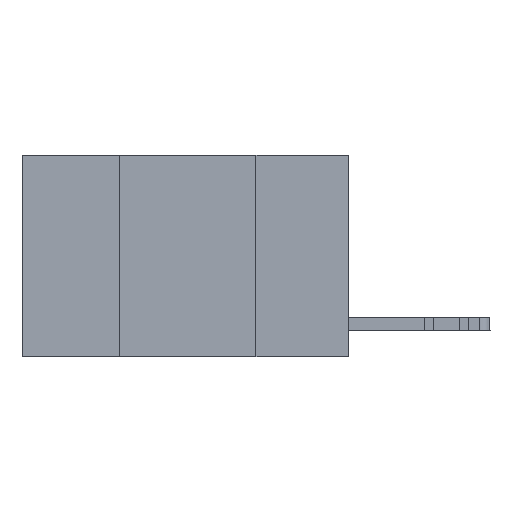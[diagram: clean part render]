
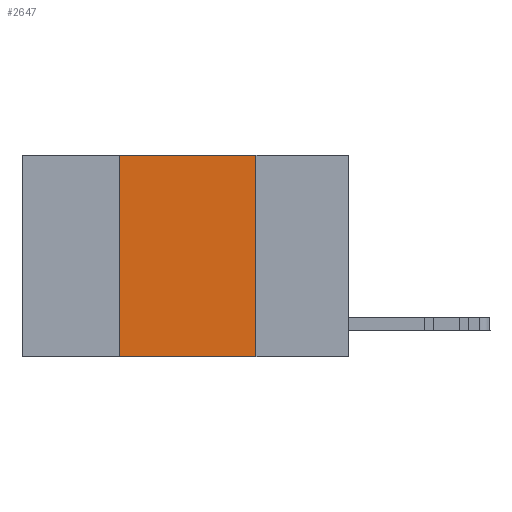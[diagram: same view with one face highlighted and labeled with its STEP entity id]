
A CAD part, left-side view. The second image highlights one B-rep face of the part: STEP entity #2647.
In plain terms, the highlighted planar face has unit normal (-1, 0, 0).
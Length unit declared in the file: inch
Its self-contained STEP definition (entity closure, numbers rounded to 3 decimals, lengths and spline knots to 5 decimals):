
#176 = PLANE ( 'NONE',  #8069 ) ;
#1855 = CARTESIAN_POINT ( 'NONE',  ( 0., 0.17, 0. ) ) ;
#2530 = CARTESIAN_POINT ( 'NONE',  ( 0., 0.6, 0. ) ) ;
#2647 = ADVANCED_FACE ( 'NONE', ( #24668 ), #176, .F. ) ;
#3897 = ORIENTED_EDGE ( 'NONE', *, *, #20488, .F. ) ;
#4731 = DIRECTION ( 'NONE',  ( 1., 0., 0. ) ) ;
#4996 = ORIENTED_EDGE ( 'NONE', *, *, #9708, .F. ) ;
#5467 = VECTOR ( 'NONE', #11132, 39.37008 ) ;
#7430 = VERTEX_POINT ( 'NONE', #26797 ) ;
#8069 = AXIS2_PLACEMENT_3D ( 'NONE', #2530, #4731, #24822 ) ;
#8283 = LINE ( 'NONE', #1855, #28602 ) ;
#8709 = DIRECTION ( 'NONE',  ( 0., 0., -1. ) ) ;
#9119 = VECTOR ( 'NONE', #28065, 39.37008 ) ;
#9708 = EDGE_CURVE ( 'NONE', #13549, #7430, #8283, .T. ) ;
#9821 = LINE ( 'NONE', #14484, #9119 ) ;
#10355 = CARTESIAN_POINT ( 'NONE',  ( 0., 0.42, 0. ) ) ;
#10970 = VERTEX_POINT ( 'NONE', #10355 ) ;
#11132 = DIRECTION ( 'NONE',  ( 0., 0., 1. ) ) ;
#11523 = VECTOR ( 'NONE', #23110, 39.37008 ) ;
#13015 = CARTESIAN_POINT ( 'NONE',  ( 0., 0.42, -0.37 ) ) ;
#13306 = ORIENTED_EDGE ( 'NONE', *, *, #21568, .F. ) ;
#13549 = VERTEX_POINT ( 'NONE', #19161 ) ;
#14484 = CARTESIAN_POINT ( 'NONE',  ( 0., 0.6, 0. ) ) ;
#14525 = LINE ( 'NONE', #16596, #11523 ) ;
#16596 = CARTESIAN_POINT ( 'NONE',  ( 0., 0.6, -0.37 ) ) ;
#19161 = CARTESIAN_POINT ( 'NONE',  ( 0., 0.17, 0. ) ) ;
#20384 = CARTESIAN_POINT ( 'NONE',  ( 0., 0.42, 0. ) ) ;
#20488 = EDGE_CURVE ( 'NONE', #10970, #13549, #9821, .T. ) ;
#20656 = EDGE_LOOP ( 'NONE', ( #4996, #3897, #13306, #23872 ) ) ;
#21568 = EDGE_CURVE ( 'NONE', #25428, #10970, #22786, .T. ) ;
#22786 = LINE ( 'NONE', #20384, #5467 ) ;
#23110 = DIRECTION ( 'NONE',  ( 0., -1., 0. ) ) ;
#23872 = ORIENTED_EDGE ( 'NONE', *, *, #27380, .T. ) ;
#24668 = FACE_OUTER_BOUND ( 'NONE', #20656, .T. ) ;
#24822 = DIRECTION ( 'NONE',  ( 0., 0., -1. ) ) ;
#25428 = VERTEX_POINT ( 'NONE', #13015 ) ;
#26797 = CARTESIAN_POINT ( 'NONE',  ( 0., 0.17, -0.37 ) ) ;
#27380 = EDGE_CURVE ( 'NONE', #25428, #7430, #14525, .T. ) ;
#28065 = DIRECTION ( 'NONE',  ( 0., -1., 0. ) ) ;
#28602 = VECTOR ( 'NONE', #8709, 39.37008 ) ;
